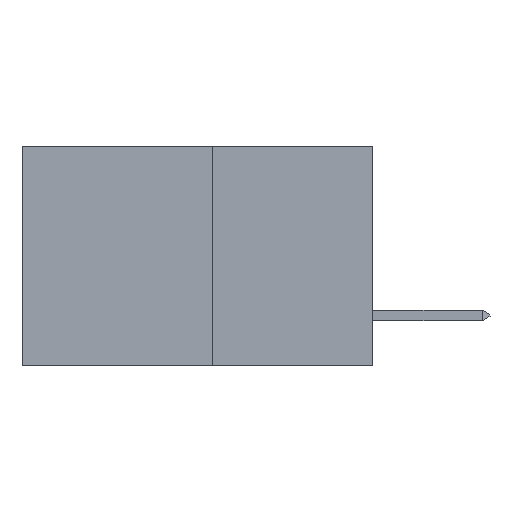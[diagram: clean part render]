
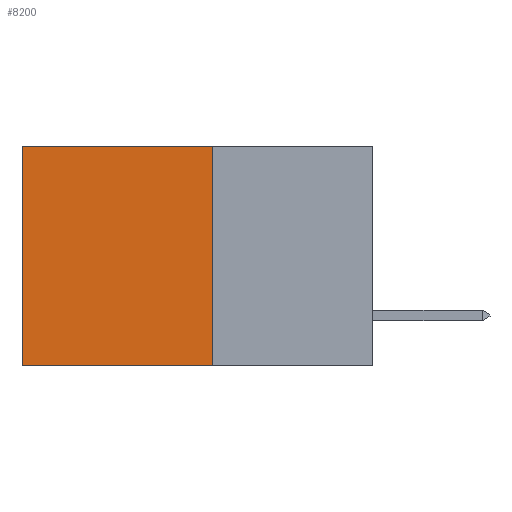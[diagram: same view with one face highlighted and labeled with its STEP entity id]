
A CAD part, left-side view. The second image highlights one B-rep face of the part: STEP entity #8200.
In plain terms, the highlighted planar face has unit normal (-1, 0, 0).
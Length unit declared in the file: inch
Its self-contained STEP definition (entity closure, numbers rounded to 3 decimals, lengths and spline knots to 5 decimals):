
#22 = DIRECTION ( 'NONE',  ( 0., 0., -1. ) ) ;
#892 = VECTOR ( 'NONE', #6627, 39.37008 ) ;
#1220 = CARTESIAN_POINT ( 'NONE',  ( 0.277, 0.27, -0.37 ) ) ;
#1787 = EDGE_CURVE ( 'NONE', #3520, #7741, #2785, .T. ) ;
#1792 = LINE ( 'NONE', #6401, #8148 ) ;
#1821 = CARTESIAN_POINT ( 'NONE',  ( 0.277, 0.27, 0. ) ) ;
#2270 = EDGE_CURVE ( 'NONE', #5917, #3757, #4745, .T. ) ;
#2696 = LINE ( 'NONE', #6902, #892 ) ;
#2785 = LINE ( 'NONE', #6011, #7620 ) ;
#3113 = FACE_OUTER_BOUND ( 'NONE', #7268, .T. ) ;
#3186 = CARTESIAN_POINT ( 'NONE',  ( 0.277, 0.27, -0.37 ) ) ;
#3239 = CARTESIAN_POINT ( 'NONE',  ( 0.277, 0.59, 0. ) ) ;
#3520 = VERTEX_POINT ( 'NONE', #3239 ) ;
#3664 = CARTESIAN_POINT ( 'NONE',  ( 0.277, 0.59, -0.37 ) ) ;
#3757 = VERTEX_POINT ( 'NONE', #4218 ) ;
#4218 = CARTESIAN_POINT ( 'NONE',  ( 0.277, 0.27, -0.37 ) ) ;
#4389 = AXIS2_PLACEMENT_3D ( 'NONE', #1220, #6250, #6036 ) ;
#4701 = ORIENTED_EDGE ( 'NONE', *, *, #7059, .F. ) ;
#4745 = LINE ( 'NONE', #3186, #7798 ) ;
#5917 = VERTEX_POINT ( 'NONE', #1821 ) ;
#6011 = CARTESIAN_POINT ( 'NONE',  ( 0.277, 0.59, -0.37 ) ) ;
#6036 = DIRECTION ( 'NONE',  ( 0., 0., -1. ) ) ;
#6087 = DIRECTION ( 'NONE',  ( 0., 0., -1. ) ) ;
#6250 = DIRECTION ( 'NONE',  ( 1., 0., 0. ) ) ;
#6401 = CARTESIAN_POINT ( 'NONE',  ( 0.277, 0.27, 0. ) ) ;
#6509 = DIRECTION ( 'NONE',  ( 0., 1., 0. ) ) ;
#6627 = DIRECTION ( 'NONE',  ( 0., 1., 0. ) ) ;
#6902 = CARTESIAN_POINT ( 'NONE',  ( 0.277, 0.27, -0.37 ) ) ;
#7059 = EDGE_CURVE ( 'NONE', #3757, #7741, #2696, .T. ) ;
#7118 = ORIENTED_EDGE ( 'NONE', *, *, #7746, .T. ) ;
#7169 = PLANE ( 'NONE',  #4389 ) ;
#7268 = EDGE_LOOP ( 'NONE', ( #8037, #4701, #8150, #7118 ) ) ;
#7620 = VECTOR ( 'NONE', #6087, 39.37008 ) ;
#7741 = VERTEX_POINT ( 'NONE', #3664 ) ;
#7746 = EDGE_CURVE ( 'NONE', #5917, #3520, #1792, .T. ) ;
#7798 = VECTOR ( 'NONE', #22, 39.37008 ) ;
#8037 = ORIENTED_EDGE ( 'NONE', *, *, #1787, .T. ) ;
#8148 = VECTOR ( 'NONE', #6509, 39.37008 ) ;
#8150 = ORIENTED_EDGE ( 'NONE', *, *, #2270, .F. ) ;
#8200 = ADVANCED_FACE ( 'NONE', ( #3113 ), #7169, .F. ) ;
